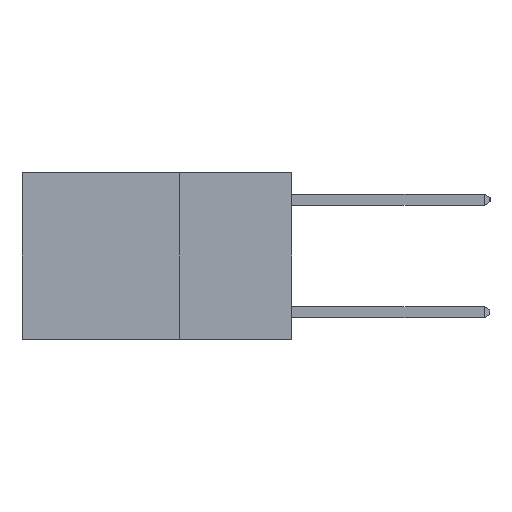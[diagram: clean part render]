
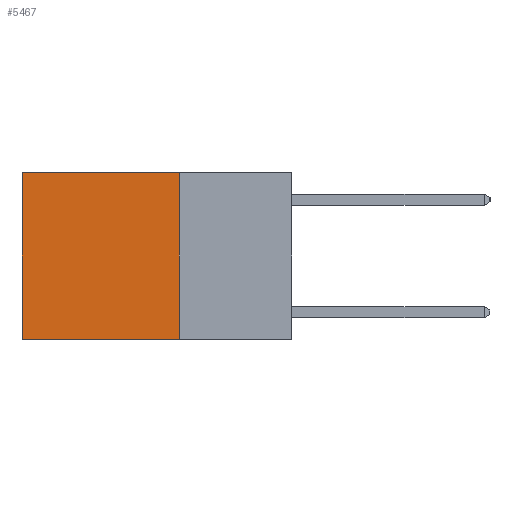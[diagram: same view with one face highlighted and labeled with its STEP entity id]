
A CAD part, left-side view. The second image highlights one B-rep face of the part: STEP entity #5467.
In plain terms, the highlighted planar face has unit normal (-1, 0, 0).
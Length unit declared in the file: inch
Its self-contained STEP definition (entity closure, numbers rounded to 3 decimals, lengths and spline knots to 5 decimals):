
#108 = VECTOR ( 'NONE', #2868, 39.37008 ) ;
#157 = VERTEX_POINT ( 'NONE', #2731 ) ;
#1027 = EDGE_CURVE ( 'NONE', #5019, #5416, #2516, .T. ) ;
#1226 = DIRECTION ( 'NONE',  ( 1., 0., 0. ) ) ;
#1382 = ORIENTED_EDGE ( 'NONE', *, *, #1826, .T. ) ;
#1647 = VECTOR ( 'NONE', #3184, 39.37008 ) ;
#1653 = ORIENTED_EDGE ( 'NONE', *, *, #6094, .F. ) ;
#1826 = EDGE_CURVE ( 'NONE', #157, #5019, #3047, .T. ) ;
#1924 = EDGE_CURVE ( 'NONE', #5665, #5416, #6616, .T. ) ;
#2516 = LINE ( 'NONE', #5882, #108 ) ;
#2590 = VECTOR ( 'NONE', #8256, 39.37008 ) ;
#2731 = CARTESIAN_POINT ( 'NONE',  ( 0.2625, 0.25, 0. ) ) ;
#2868 = DIRECTION ( 'NONE',  ( 0., 0., -1. ) ) ;
#3043 = AXIS2_PLACEMENT_3D ( 'NONE', #9815, #1226, #7385 ) ;
#3047 = LINE ( 'NONE', #10221, #9597 ) ;
#3096 = CARTESIAN_POINT ( 'NONE',  ( 0.2625, 0.6, 0. ) ) ;
#3184 = DIRECTION ( 'NONE',  ( 0., 1., 0. ) ) ;
#3721 = CARTESIAN_POINT ( 'NONE',  ( 0.2625, 0.25, -0.37 ) ) ;
#4693 = FACE_OUTER_BOUND ( 'NONE', #10714, .T. ) ;
#5019 = VERTEX_POINT ( 'NONE', #3096 ) ;
#5416 = VERTEX_POINT ( 'NONE', #6425 ) ;
#5467 = ADVANCED_FACE ( 'NONE', ( #4693 ), #10580, .F. ) ;
#5665 = VERTEX_POINT ( 'NONE', #8449 ) ;
#5882 = CARTESIAN_POINT ( 'NONE',  ( 0.2625, 0.6, 0. ) ) ;
#6094 = EDGE_CURVE ( 'NONE', #157, #5665, #7258, .T. ) ;
#6425 = CARTESIAN_POINT ( 'NONE',  ( 0.2625, 0.6, -0.37 ) ) ;
#6616 = LINE ( 'NONE', #3721, #1647 ) ;
#7258 = LINE ( 'NONE', #10641, #2590 ) ;
#7385 = DIRECTION ( 'NONE',  ( 0., 0., -1. ) ) ;
#8256 = DIRECTION ( 'NONE',  ( 0., 0., -1. ) ) ;
#8449 = CARTESIAN_POINT ( 'NONE',  ( 0.2625, 0.25, -0.37 ) ) ;
#8573 = ORIENTED_EDGE ( 'NONE', *, *, #1924, .F. ) ;
#9505 = DIRECTION ( 'NONE',  ( 0., 1., 0. ) ) ;
#9597 = VECTOR ( 'NONE', #9505, 39.37008 ) ;
#9815 = CARTESIAN_POINT ( 'NONE',  ( 0.2625, 0.25, 0. ) ) ;
#10221 = CARTESIAN_POINT ( 'NONE',  ( 0.2625, 0.25, 0. ) ) ;
#10580 = PLANE ( 'NONE',  #3043 ) ;
#10641 = CARTESIAN_POINT ( 'NONE',  ( 0.2625, 0.25, 0. ) ) ;
#10701 = ORIENTED_EDGE ( 'NONE', *, *, #1027, .T. ) ;
#10714 = EDGE_LOOP ( 'NONE', ( #10701, #8573, #1653, #1382 ) ) ;
